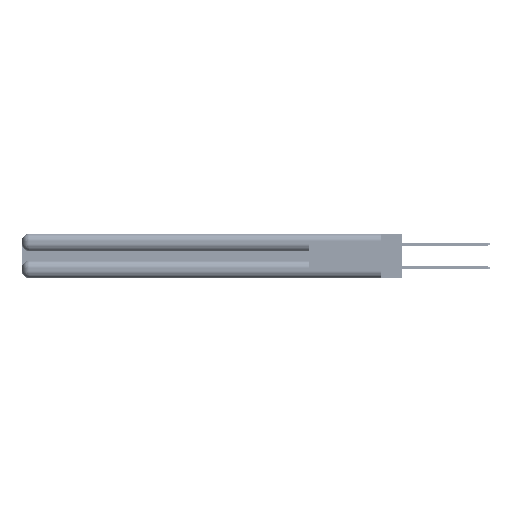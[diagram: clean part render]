
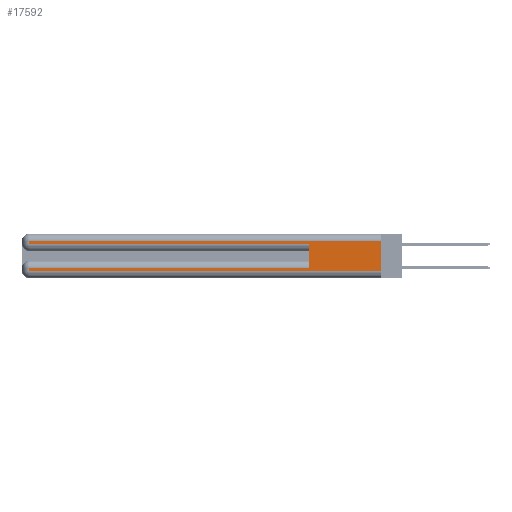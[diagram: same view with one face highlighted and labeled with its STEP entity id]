
A CAD part, left-side view. The second image highlights one B-rep face of the part: STEP entity #17592.
In plain terms, the highlighted planar face has unit normal (-1, 0, 0).
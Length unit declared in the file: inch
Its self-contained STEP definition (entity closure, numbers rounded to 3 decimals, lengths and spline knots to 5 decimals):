
#1360 = EDGE_CURVE ( 'NONE', #4485, #21739, #24395, .T. ) ;
#3615 = CARTESIAN_POINT ( 'NONE',  ( 0., 0., 0.31 ) ) ;
#4485 = VERTEX_POINT ( 'NONE', #6999 ) ;
#4525 = FACE_OUTER_BOUND ( 'NONE', #5736, .T. ) ;
#4771 = LINE ( 'NONE', #54134, #26465 ) ;
#5110 = DIRECTION ( 'NONE',  ( 1., 0., 0. ) ) ;
#5736 = EDGE_LOOP ( 'NONE', ( #11890, #37533, #54261, #13280, #49709, #37689, #10041, #28236 ) ) ;
#6888 = DIRECTION ( 'NONE',  ( 0., 0., -1. ) ) ;
#6999 = CARTESIAN_POINT ( 'NONE',  ( 0., 0.6, 0.085 ) ) ;
#7416 = CARTESIAN_POINT ( 'NONE',  ( 0., 0.6, 0.285 ) ) ;
#8341 = VECTOR ( 'NONE', #18208, 39.37008 ) ;
#8550 = CARTESIAN_POINT ( 'NONE',  ( 0., 0., 0.06 ) ) ;
#9422 = EDGE_CURVE ( 'NONE', #4485, #39451, #47515, .T. ) ;
#10041 = ORIENTED_EDGE ( 'NONE', *, *, #28285, .T. ) ;
#10718 = CARTESIAN_POINT ( 'NONE',  ( 0., 2.94, 0.085 ) ) ;
#11428 = CARTESIAN_POINT ( 'NONE',  ( 0., 2.94, 0.37 ) ) ;
#11602 = EDGE_CURVE ( 'NONE', #12611, #41048, #53976, .T. ) ;
#11890 = ORIENTED_EDGE ( 'NONE', *, *, #11602, .F. ) ;
#12611 = VERTEX_POINT ( 'NONE', #3615 ) ;
#12877 = VECTOR ( 'NONE', #20264, 39.37008 ) ;
#13280 = ORIENTED_EDGE ( 'NONE', *, *, #31805, .T. ) ;
#13880 = CARTESIAN_POINT ( 'NONE',  ( 0., 0., 0.37 ) ) ;
#15925 = VECTOR ( 'NONE', #53189, 39.37008 ) ;
#17592 = ADVANCED_FACE ( 'NONE', ( #4525 ), #18234, .F. ) ;
#17977 = DIRECTION ( 'NONE',  ( 0., -1., 0. ) ) ;
#18208 = DIRECTION ( 'NONE',  ( 0., 1., 0. ) ) ;
#18234 = PLANE ( 'NONE',  #24845 ) ;
#18515 = LINE ( 'NONE', #11428, #38724 ) ;
#18745 = DIRECTION ( 'NONE',  ( 0., 0., -1. ) ) ;
#19387 = VERTEX_POINT ( 'NONE', #55422 ) ;
#19404 = VECTOR ( 'NONE', #20126, 39.37008 ) ;
#20126 = DIRECTION ( 'NONE',  ( 0., -1., 0. ) ) ;
#20264 = DIRECTION ( 'NONE',  ( 0., 0., 1. ) ) ;
#21739 = VERTEX_POINT ( 'NONE', #7416 ) ;
#22586 = DIRECTION ( 'NONE',  ( 0., 0., -1. ) ) ;
#22621 = VERTEX_POINT ( 'NONE', #43569 ) ;
#23216 = CARTESIAN_POINT ( 'NONE',  ( 0., 0., 0.085 ) ) ;
#24299 = CARTESIAN_POINT ( 'NONE',  ( 0., 0., 0.285 ) ) ;
#24395 = LINE ( 'NONE', #37398, #12877 ) ;
#24845 = AXIS2_PLACEMENT_3D ( 'NONE', #13880, #5110, #22586 ) ;
#26465 = VECTOR ( 'NONE', #6888, 39.37008 ) ;
#27124 = EDGE_CURVE ( 'NONE', #12611, #46837, #50121, .T. ) ;
#28236 = ORIENTED_EDGE ( 'NONE', *, *, #44799, .T. ) ;
#28285 = EDGE_CURVE ( 'NONE', #39451, #19387, #4771, .T. ) ;
#30257 = CARTESIAN_POINT ( 'NONE',  ( 0., 0., 0.31 ) ) ;
#31154 = VECTOR ( 'NONE', #18745, 39.37008 ) ;
#31805 = EDGE_CURVE ( 'NONE', #22621, #21739, #53657, .T. ) ;
#31930 = VECTOR ( 'NONE', #17977, 39.37008 ) ;
#34632 = LINE ( 'NONE', #52322, #31930 ) ;
#37398 = CARTESIAN_POINT ( 'NONE',  ( 0., 0.6, 0.145 ) ) ;
#37533 = ORIENTED_EDGE ( 'NONE', *, *, #27124, .T. ) ;
#37689 = ORIENTED_EDGE ( 'NONE', *, *, #9422, .T. ) ;
#38724 = VECTOR ( 'NONE', #41552, 39.37008 ) ;
#39451 = VERTEX_POINT ( 'NONE', #10718 ) ;
#40204 = CARTESIAN_POINT ( 'NONE',  ( 0., 0., 0.37 ) ) ;
#41048 = VERTEX_POINT ( 'NONE', #8550 ) ;
#41552 = DIRECTION ( 'NONE',  ( 0., 0., -1. ) ) ;
#43569 = CARTESIAN_POINT ( 'NONE',  ( 0., 2.94, 0.285 ) ) ;
#44799 = EDGE_CURVE ( 'NONE', #19387, #41048, #34632, .T. ) ;
#46837 = VERTEX_POINT ( 'NONE', #51288 ) ;
#47515 = LINE ( 'NONE', #23216, #15925 ) ;
#49067 = EDGE_CURVE ( 'NONE', #46837, #22621, #18515, .T. ) ;
#49709 = ORIENTED_EDGE ( 'NONE', *, *, #1360, .F. ) ;
#50121 = LINE ( 'NONE', #30257, #8341 ) ;
#51288 = CARTESIAN_POINT ( 'NONE',  ( 0., 2.94, 0.31 ) ) ;
#52322 = CARTESIAN_POINT ( 'NONE',  ( 0., 0., 0.06 ) ) ;
#53189 = DIRECTION ( 'NONE',  ( 0., 1., 0. ) ) ;
#53657 = LINE ( 'NONE', #24299, #19404 ) ;
#53976 = LINE ( 'NONE', #40204, #31154 ) ;
#54134 = CARTESIAN_POINT ( 'NONE',  ( 0., 2.94, 0.37 ) ) ;
#54261 = ORIENTED_EDGE ( 'NONE', *, *, #49067, .T. ) ;
#55422 = CARTESIAN_POINT ( 'NONE',  ( 0., 2.94, 0.06 ) ) ;
